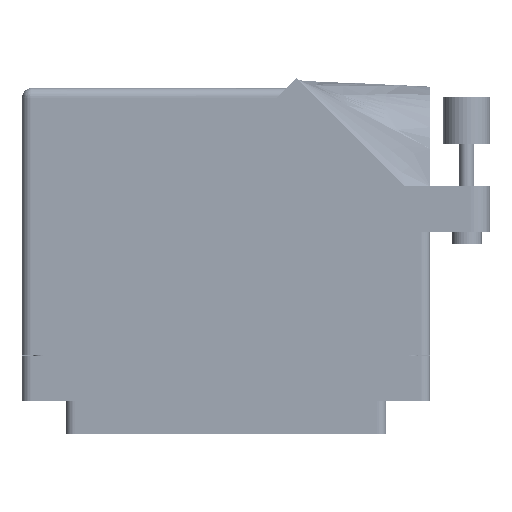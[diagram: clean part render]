
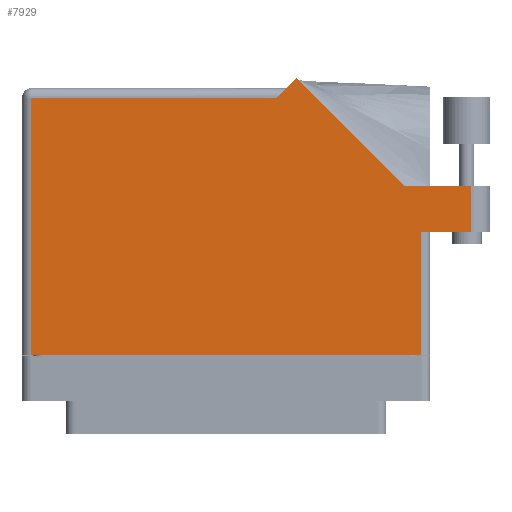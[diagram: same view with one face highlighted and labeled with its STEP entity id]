
A CAD part, front view. The second image highlights one B-rep face of the part: STEP entity #7929.
In plain terms, the highlighted face is planar.
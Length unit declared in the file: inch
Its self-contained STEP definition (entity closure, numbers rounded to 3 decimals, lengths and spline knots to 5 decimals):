
#601 = ORIENTED_EDGE ( 'NONE', *, *, #51599, .T. ) ;
#894 = VERTEX_POINT ( 'NONE', #36865 ) ;
#3596 = VECTOR ( 'NONE', #17477, 39.37008 ) ;
#4890 = CARTESIAN_POINT ( 'NONE',  ( 1.634, 1.022, 0.617 ) ) ;
#5270 = LINE ( 'NONE', #69319, #45935 ) ;
#5374 = CARTESIAN_POINT ( 'NONE',  ( 1.759, 1.022, 0.617 ) ) ;
#6130 = CARTESIAN_POINT ( 'NONE',  ( -1.359, 1.675, 0.617 ) ) ;
#6764 = CARTESIAN_POINT ( 'NONE',  ( 1.297, -0.1, 0.617 ) ) ;
#7929 = ADVANCED_FACE ( 'NONE', ( #66606 ), #34583, .F. ) ;
#8297 = VECTOR ( 'NONE', #9907, 39.37008 ) ;
#8393 = CARTESIAN_POINT ( 'NONE',  ( 1.359, 0.715, 0.617 ) ) ;
#9907 = DIRECTION ( 'NONE',  ( 0., 1., 0. ) ) ;
#10459 = CARTESIAN_POINT ( 'NONE',  ( 1.297, 0.715, 0.617 ) ) ;
#12185 = DIRECTION ( 'NONE',  ( -1., 0., 0. ) ) ;
#12912 = VERTEX_POINT ( 'NONE', #16617 ) ;
#13037 = CARTESIAN_POINT ( 'NONE',  ( -1.297, -0.1, 0.617 ) ) ;
#13993 = VECTOR ( 'NONE', #61059, 39.37008 ) ;
#13996 = VERTEX_POINT ( 'NONE', #44534 ) ;
#16534 = CARTESIAN_POINT ( 'NONE',  ( -1.359, 1.613, 0.617 ) ) ;
#16617 = CARTESIAN_POINT ( 'NONE',  ( -1.297, -0.1, 0.617 ) ) ;
#17303 = LINE ( 'NONE', #13037, #13993 ) ;
#17477 = DIRECTION ( 'NONE',  ( -0.707, 0.707, 0. ) ) ;
#18748 = CARTESIAN_POINT ( 'NONE',  ( -1.297, 1.613, 0.617 ) ) ;
#18770 = VERTEX_POINT ( 'NONE', #26119 ) ;
#21151 = LINE ( 'NONE', #10459, #33710 ) ;
#23427 = EDGE_LOOP ( 'NONE', ( #25439, #61181, #45630, #32866, #39352, #57671, #53916, #48974, #601 ) ) ;
#23774 = VERTEX_POINT ( 'NONE', #57037 ) ;
#24700 = CARTESIAN_POINT ( 'NONE',  ( -1.359, -0.1, 0.617 ) ) ;
#24924 = VERTEX_POINT ( 'NONE', #54687 ) ;
#25439 = ORIENTED_EDGE ( 'NONE', *, *, #67183, .T. ) ;
#26119 = CARTESIAN_POINT ( 'NONE',  ( 1.634, 1.022, 0.617 ) ) ;
#26743 = LINE ( 'NONE', #5374, #57411 ) ;
#27568 = LINE ( 'NONE', #16534, #31130 ) ;
#28581 = EDGE_CURVE ( 'NONE', #41725, #12912, #17303, .T. ) ;
#28872 = LINE ( 'NONE', #33514, #3596 ) ;
#28898 = EDGE_CURVE ( 'NONE', #23774, #41725, #27568, .T. ) ;
#31130 = VECTOR ( 'NONE', #58879, 39.37008 ) ;
#31190 = VERTEX_POINT ( 'NONE', #6764 ) ;
#32866 = ORIENTED_EDGE ( 'NONE', *, *, #70285, .T. ) ;
#33278 = VERTEX_POINT ( 'NONE', #50683 ) ;
#33514 = CARTESIAN_POINT ( 'NONE',  ( 1.19342, 1.022, 0.617 ) ) ;
#33710 = VECTOR ( 'NONE', #49205, 39.37008 ) ;
#34583 = PLANE ( 'NONE',  #62169 ) ;
#36865 = CARTESIAN_POINT ( 'NONE',  ( 1.634, 0.715, 0.617 ) ) ;
#39352 = ORIENTED_EDGE ( 'NONE', *, *, #49444, .T. ) ;
#39974 = LINE ( 'NONE', #24700, #65591 ) ;
#41725 = VERTEX_POINT ( 'NONE', #18748 ) ;
#42269 = DIRECTION ( 'NONE',  ( -0.707, -0.707, 0. ) ) ;
#42829 = VECTOR ( 'NONE', #67104, 39.37008 ) ;
#44534 = CARTESIAN_POINT ( 'NONE',  ( 1.297, 0.715, 0.617 ) ) ;
#45397 = LINE ( 'NONE', #8393, #42829 ) ;
#45630 = ORIENTED_EDGE ( 'NONE', *, *, #50853, .T. ) ;
#45935 = VECTOR ( 'NONE', #42269, 39.37008 ) ;
#48974 = ORIENTED_EDGE ( 'NONE', *, *, #67580, .T. ) ;
#49205 = DIRECTION ( 'NONE',  ( 0., 1., 0. ) ) ;
#49444 = EDGE_CURVE ( 'NONE', #24924, #23774, #5270, .T. ) ;
#50060 = DIRECTION ( 'NONE',  ( -1., 0., 0. ) ) ;
#50683 = CARTESIAN_POINT ( 'NONE',  ( 1.19342, 1.022, 0.617 ) ) ;
#50853 = EDGE_CURVE ( 'NONE', #18770, #33278, #26743, .T. ) ;
#51599 = EDGE_CURVE ( 'NONE', #31190, #13996, #21151, .T. ) ;
#53916 = ORIENTED_EDGE ( 'NONE', *, *, #28581, .T. ) ;
#54687 = CARTESIAN_POINT ( 'NONE',  ( 0.46971, 1.74571, 0.617 ) ) ;
#57037 = CARTESIAN_POINT ( 'NONE',  ( 0.337, 1.613, 0.617 ) ) ;
#57411 = VECTOR ( 'NONE', #50060, 39.37008 ) ;
#57671 = ORIENTED_EDGE ( 'NONE', *, *, #28898, .T. ) ;
#58618 = LINE ( 'NONE', #4890, #8297 ) ;
#58879 = DIRECTION ( 'NONE',  ( -1., 0., 0. ) ) ;
#60189 = DIRECTION ( 'NONE',  ( 0., 0., -1. ) ) ;
#61059 = DIRECTION ( 'NONE',  ( 0., -1., 0. ) ) ;
#61181 = ORIENTED_EDGE ( 'NONE', *, *, #61637, .T. ) ;
#61308 = DIRECTION ( 'NONE',  ( 1., 0., 0. ) ) ;
#61637 = EDGE_CURVE ( 'NONE', #894, #18770, #58618, .T. ) ;
#62169 = AXIS2_PLACEMENT_3D ( 'NONE', #6130, #60189, #12185 ) ;
#65591 = VECTOR ( 'NONE', #61308, 39.37008 ) ;
#66606 = FACE_OUTER_BOUND ( 'NONE', #23427, .T. ) ;
#67104 = DIRECTION ( 'NONE',  ( 1., 0., 0. ) ) ;
#67183 = EDGE_CURVE ( 'NONE', #13996, #894, #45397, .T. ) ;
#67580 = EDGE_CURVE ( 'NONE', #12912, #31190, #39974, .T. ) ;
#69319 = CARTESIAN_POINT ( 'NONE',  ( 0.399, 1.675, 0.617 ) ) ;
#70285 = EDGE_CURVE ( 'NONE', #33278, #24924, #28872, .T. ) ;
